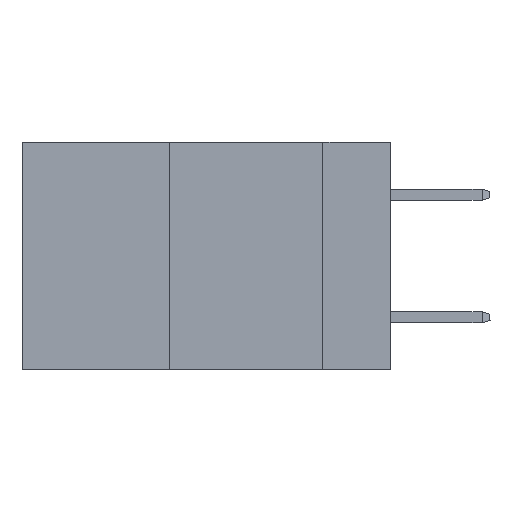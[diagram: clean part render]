
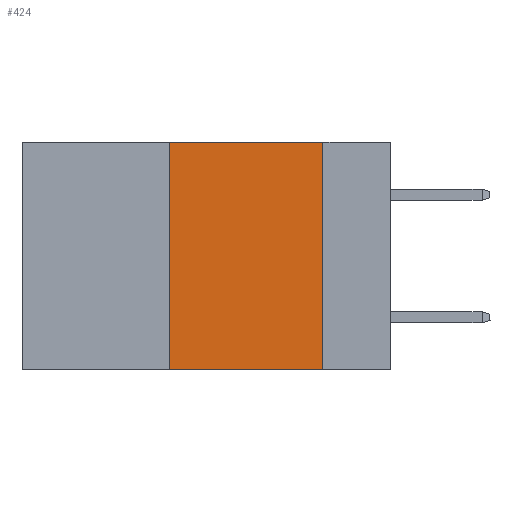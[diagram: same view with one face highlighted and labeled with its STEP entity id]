
A CAD part, left-side view. The second image highlights one B-rep face of the part: STEP entity #424.
In plain terms, the highlighted planar face has unit normal (-1, 0, 0).
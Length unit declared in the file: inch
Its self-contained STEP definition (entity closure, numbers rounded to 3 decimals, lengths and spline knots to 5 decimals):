
#110 = DIRECTION ( 'NONE',  ( 1., 0., 0. ) ) ;
#339 = VECTOR ( 'NONE', #11842, 39.37008 ) ;
#424 = ADVANCED_FACE ( 'NONE', ( #6249 ), #12677, .F. ) ;
#2715 = CARTESIAN_POINT ( 'NONE',  ( 0., 0.11, -0.37 ) ) ;
#2747 = AXIS2_PLACEMENT_3D ( 'NONE', #16126, #110, #16379 ) ;
#3791 = DIRECTION ( 'NONE',  ( 0., 0., 1. ) ) ;
#4260 = CARTESIAN_POINT ( 'NONE',  ( 0., 0.6, -0.37 ) ) ;
#4380 = VECTOR ( 'NONE', #19656, 39.37008 ) ;
#4443 = LINE ( 'NONE', #12471, #5254 ) ;
#4997 = CARTESIAN_POINT ( 'NONE',  ( 0., 0.11, 0. ) ) ;
#5202 = VERTEX_POINT ( 'NONE', #4997 ) ;
#5254 = VECTOR ( 'NONE', #3791, 39.37008 ) ;
#6249 = FACE_OUTER_BOUND ( 'NONE', #14861, .T. ) ;
#6278 = LINE ( 'NONE', #8553, #9887 ) ;
#7100 = CARTESIAN_POINT ( 'NONE',  ( 0., 0.11, 0. ) ) ;
#8553 = CARTESIAN_POINT ( 'NONE',  ( 0., 0.6, 0. ) ) ;
#8647 = ORIENTED_EDGE ( 'NONE', *, *, #16944, .T. ) ;
#8879 = CARTESIAN_POINT ( 'NONE',  ( 0., 0.36, 0. ) ) ;
#9887 = VECTOR ( 'NONE', #12981, 39.37008 ) ;
#9915 = LINE ( 'NONE', #4260, #339 ) ;
#10965 = CARTESIAN_POINT ( 'NONE',  ( 0., 0.36, -0.37 ) ) ;
#11128 = ORIENTED_EDGE ( 'NONE', *, *, #20749, .F. ) ;
#11670 = ORIENTED_EDGE ( 'NONE', *, *, #15650, .F. ) ;
#11842 = DIRECTION ( 'NONE',  ( 0., -1., 0. ) ) ;
#12471 = CARTESIAN_POINT ( 'NONE',  ( 0., 0.36, 0. ) ) ;
#12677 = PLANE ( 'NONE',  #2747 ) ;
#12981 = DIRECTION ( 'NONE',  ( 0., -1., 0. ) ) ;
#13566 = VERTEX_POINT ( 'NONE', #8879 ) ;
#14861 = EDGE_LOOP ( 'NONE', ( #11670, #18073, #11128, #8647 ) ) ;
#15650 = EDGE_CURVE ( 'NONE', #5202, #20553, #20726, .T. ) ;
#16126 = CARTESIAN_POINT ( 'NONE',  ( 0., 0.6, 0. ) ) ;
#16379 = DIRECTION ( 'NONE',  ( 0., 0., -1. ) ) ;
#16944 = EDGE_CURVE ( 'NONE', #17608, #20553, #9915, .T. ) ;
#17334 = EDGE_CURVE ( 'NONE', #13566, #5202, #6278, .T. ) ;
#17608 = VERTEX_POINT ( 'NONE', #10965 ) ;
#18073 = ORIENTED_EDGE ( 'NONE', *, *, #17334, .F. ) ;
#19656 = DIRECTION ( 'NONE',  ( 0., 0., -1. ) ) ;
#20553 = VERTEX_POINT ( 'NONE', #2715 ) ;
#20726 = LINE ( 'NONE', #7100, #4380 ) ;
#20749 = EDGE_CURVE ( 'NONE', #17608, #13566, #4443, .T. ) ;
